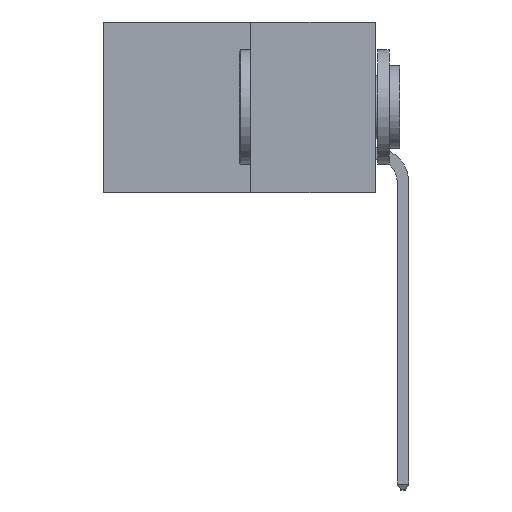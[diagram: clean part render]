
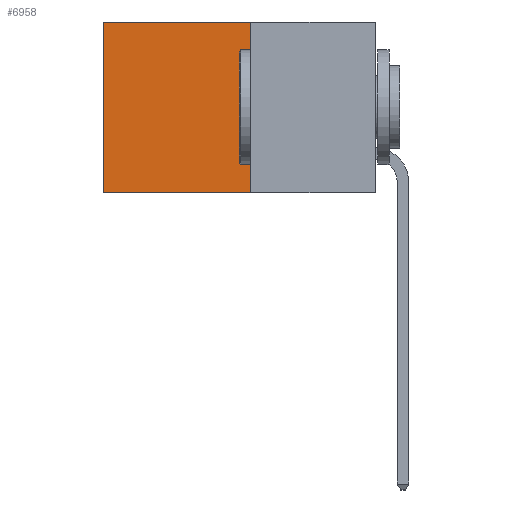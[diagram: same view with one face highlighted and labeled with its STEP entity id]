
A CAD part, left-side view. The second image highlights one B-rep face of the part: STEP entity #6958.
In plain terms, the highlighted planar face has unit normal (-1, 0, 0).
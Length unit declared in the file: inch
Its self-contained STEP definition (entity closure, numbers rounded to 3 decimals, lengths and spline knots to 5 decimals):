
#380 = LINE ( 'NONE', #12184, #11182 ) ;
#1419 = DIRECTION ( 'NONE',  ( 0., 1., 0. ) ) ;
#1596 = DIRECTION ( 'NONE',  ( 0., 1., 0. ) ) ;
#2040 = EDGE_CURVE ( 'NONE', #6970, #20745, #9415, .T. ) ;
#3227 = CARTESIAN_POINT ( 'NONE',  ( 0.277, 0.59, -0.37 ) ) ;
#4305 = ORIENTED_EDGE ( 'NONE', *, *, #2040, .F. ) ;
#5234 = AXIS2_PLACEMENT_3D ( 'NONE', #6700, #21629, #8845 ) ;
#5417 = DIRECTION ( 'NONE',  ( 0., 0., -1. ) ) ;
#6700 = CARTESIAN_POINT ( 'NONE',  ( 0.277, 0.27, -0.37 ) ) ;
#6827 = VECTOR ( 'NONE', #5417, 39.37008 ) ;
#6958 = ADVANCED_FACE ( 'NONE', ( #22472 ), #17382, .F. ) ;
#6970 = VERTEX_POINT ( 'NONE', #19596 ) ;
#7943 = CARTESIAN_POINT ( 'NONE',  ( 0.277, 0.27, -0.37 ) ) ;
#8845 = DIRECTION ( 'NONE',  ( 0., 0., -1. ) ) ;
#9415 = LINE ( 'NONE', #22198, #25757 ) ;
#9516 = CARTESIAN_POINT ( 'NONE',  ( 0.277, 0.59, 0. ) ) ;
#11182 = VECTOR ( 'NONE', #1419, 39.37008 ) ;
#11996 = VERTEX_POINT ( 'NONE', #9516 ) ;
#12184 = CARTESIAN_POINT ( 'NONE',  ( 0.277, 0.27, -0.37 ) ) ;
#12359 = CARTESIAN_POINT ( 'NONE',  ( 0.277, 0.27, 0. ) ) ;
#12385 = ORIENTED_EDGE ( 'NONE', *, *, #26196, .F. ) ;
#12802 = ORIENTED_EDGE ( 'NONE', *, *, #20618, .T. ) ;
#13692 = VERTEX_POINT ( 'NONE', #26779 ) ;
#14168 = LINE ( 'NONE', #12359, #24812 ) ;
#17382 = PLANE ( 'NONE',  #5234 ) ;
#18953 = ORIENTED_EDGE ( 'NONE', *, *, #27525, .T. ) ;
#19596 = CARTESIAN_POINT ( 'NONE',  ( 0.277, 0.27, 0. ) ) ;
#20618 = EDGE_CURVE ( 'NONE', #11996, #13692, #23852, .T. ) ;
#20745 = VERTEX_POINT ( 'NONE', #7943 ) ;
#21629 = DIRECTION ( 'NONE',  ( 1., 0., 0. ) ) ;
#22103 = DIRECTION ( 'NONE',  ( 0., 0., -1. ) ) ;
#22198 = CARTESIAN_POINT ( 'NONE',  ( 0.277, 0.27, -0.37 ) ) ;
#22472 = FACE_OUTER_BOUND ( 'NONE', #24185, .T. ) ;
#23852 = LINE ( 'NONE', #3227, #6827 ) ;
#24185 = EDGE_LOOP ( 'NONE', ( #12802, #12385, #4305, #18953 ) ) ;
#24812 = VECTOR ( 'NONE', #1596, 39.37008 ) ;
#25757 = VECTOR ( 'NONE', #22103, 39.37008 ) ;
#26196 = EDGE_CURVE ( 'NONE', #20745, #13692, #380, .T. ) ;
#26779 = CARTESIAN_POINT ( 'NONE',  ( 0.277, 0.59, -0.37 ) ) ;
#27525 = EDGE_CURVE ( 'NONE', #6970, #11996, #14168, .T. ) ;
